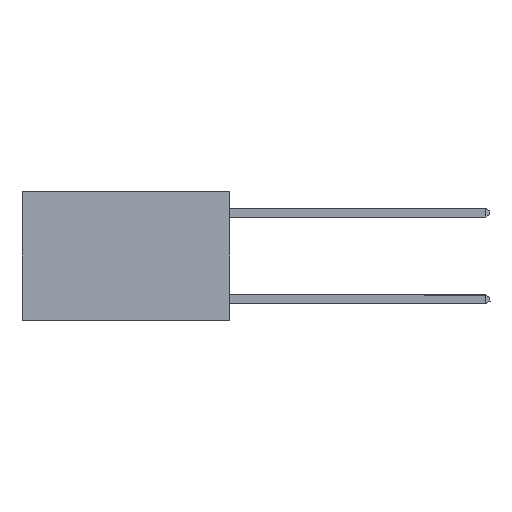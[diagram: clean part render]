
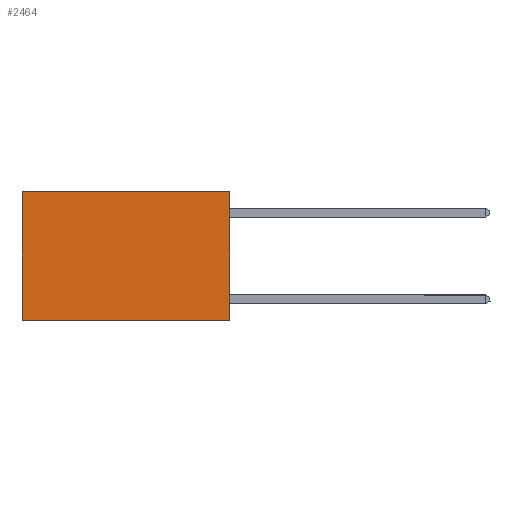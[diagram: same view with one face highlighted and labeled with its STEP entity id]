
A CAD part, left-side view. The second image highlights one B-rep face of the part: STEP entity #2464.
In plain terms, the highlighted planar face has unit normal (-1, 0, 0).
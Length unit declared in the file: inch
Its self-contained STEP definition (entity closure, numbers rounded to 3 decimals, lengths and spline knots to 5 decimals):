
#889 = ORIENTED_EDGE ( 'NONE', *, *, #13132, .F. ) ;
#2182 = VERTEX_POINT ( 'NONE', #26300 ) ;
#2464 = ADVANCED_FACE ( 'NONE', ( #11310 ), #16862, .F. ) ;
#2698 = LINE ( 'NONE', #25750, #13392 ) ;
#4838 = VERTEX_POINT ( 'NONE', #22421 ) ;
#4898 = EDGE_CURVE ( 'NONE', #24481, #2182, #20262, .T. ) ;
#5134 = LINE ( 'NONE', #13048, #26576 ) ;
#6188 = EDGE_CURVE ( 'NONE', #2182, #4838, #5134, .T. ) ;
#6582 = DIRECTION ( 'NONE',  ( 0., 0., -1. ) ) ;
#8893 = VECTOR ( 'NONE', #16188, 39.37008 ) ;
#10528 = DIRECTION ( 'NONE',  ( 1., 0., 0. ) ) ;
#11310 = FACE_OUTER_BOUND ( 'NONE', #22169, .T. ) ;
#11703 = CARTESIAN_POINT ( 'NONE',  ( 0.2625, 0., -0.37 ) ) ;
#12053 = ORIENTED_EDGE ( 'NONE', *, *, #6188, .T. ) ;
#12599 = VECTOR ( 'NONE', #21854, 39.37008 ) ;
#13048 = CARTESIAN_POINT ( 'NONE',  ( 0.2625, 0.6, 0. ) ) ;
#13132 = EDGE_CURVE ( 'NONE', #21350, #4838, #18257, .T. ) ;
#13392 = VECTOR ( 'NONE', #15043, 39.37008 ) ;
#14686 = ORIENTED_EDGE ( 'NONE', *, *, #4898, .T. ) ;
#14823 = CARTESIAN_POINT ( 'NONE',  ( 0.2625, 0., 0. ) ) ;
#15043 = DIRECTION ( 'NONE',  ( 0., 0., -1. ) ) ;
#16188 = DIRECTION ( 'NONE',  ( 0., 1., 0. ) ) ;
#16862 = PLANE ( 'NONE',  #23191 ) ;
#18257 = LINE ( 'NONE', #19666, #12599 ) ;
#19666 = CARTESIAN_POINT ( 'NONE',  ( 0.2625, 0., -0.37 ) ) ;
#20262 = LINE ( 'NONE', #22608, #8893 ) ;
#21350 = VERTEX_POINT ( 'NONE', #11703 ) ;
#21854 = DIRECTION ( 'NONE',  ( 0., 1., 0. ) ) ;
#22169 = EDGE_LOOP ( 'NONE', ( #12053, #889, #22653, #14686 ) ) ;
#22421 = CARTESIAN_POINT ( 'NONE',  ( 0.2625, 0.6, -0.37 ) ) ;
#22608 = CARTESIAN_POINT ( 'NONE',  ( 0.2625, 0., 0. ) ) ;
#22653 = ORIENTED_EDGE ( 'NONE', *, *, #23116, .F. ) ;
#23116 = EDGE_CURVE ( 'NONE', #24481, #21350, #2698, .T. ) ;
#23191 = AXIS2_PLACEMENT_3D ( 'NONE', #23371, #10528, #25523 ) ;
#23371 = CARTESIAN_POINT ( 'NONE',  ( 0.2625, 0., 0. ) ) ;
#24481 = VERTEX_POINT ( 'NONE', #14823 ) ;
#25523 = DIRECTION ( 'NONE',  ( 0., 0., -1. ) ) ;
#25750 = CARTESIAN_POINT ( 'NONE',  ( 0.2625, 0., 0. ) ) ;
#26300 = CARTESIAN_POINT ( 'NONE',  ( 0.2625, 0.6, 0. ) ) ;
#26576 = VECTOR ( 'NONE', #6582, 39.37008 ) ;
